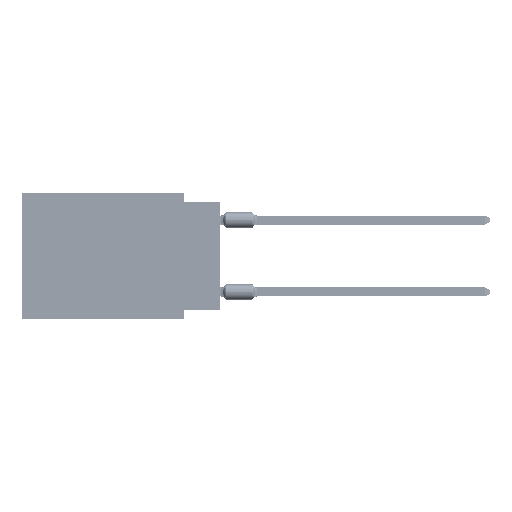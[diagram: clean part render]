
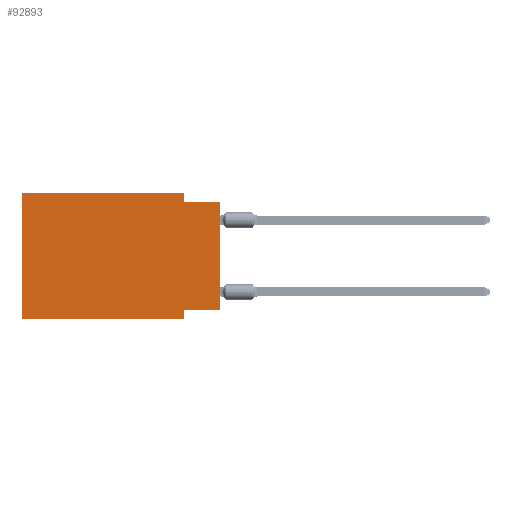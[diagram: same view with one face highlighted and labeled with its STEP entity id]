
A CAD part, left-side view. The second image highlights one B-rep face of the part: STEP entity #92893.
In plain terms, the highlighted planar face has unit normal (-1, 0, 0).
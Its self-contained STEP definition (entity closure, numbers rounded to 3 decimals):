
#2600 = CARTESIAN_POINT ( 'NONE',  ( 0., 0., -8.255 ) ) ;
#4311 = DIRECTION ( 'NONE',  ( 0., -1., 0. ) ) ;
#6535 = CARTESIAN_POINT ( 'NONE',  ( 0., 0., -0.635 ) ) ;
#6693 = CARTESIAN_POINT ( 'NONE',  ( 0., 0., 0. ) ) ;
#10922 = DIRECTION ( 'NONE',  ( 0., 0., -1. ) ) ;
#11883 = CARTESIAN_POINT ( 'NONE',  ( 0., 13.97, 0. ) ) ;
#12060 = FACE_OUTER_BOUND ( 'NONE', #67928, .T. ) ;
#13523 = DIRECTION ( 'NONE',  ( 0., 0., -1. ) ) ;
#13532 = EDGE_CURVE ( 'NONE', #15700, #110712, #107723, .T. ) ;
#14979 = LINE ( 'NONE', #6693, #100737 ) ;
#15146 = CARTESIAN_POINT ( 'NONE',  ( 0., 13.97, -8.89 ) ) ;
#15330 = CARTESIAN_POINT ( 'NONE',  ( 0., 2.54, -0.635 ) ) ;
#15700 = VERTEX_POINT ( 'NONE', #2600 ) ;
#16243 = CARTESIAN_POINT ( 'NONE',  ( 0., 0., -0.635 ) ) ;
#17698 = DIRECTION ( 'NONE',  ( 0., 1., 0. ) ) ;
#19477 = EDGE_CURVE ( 'NONE', #15700, #97066, #14979, .T. ) ;
#24214 = ORIENTED_EDGE ( 'NONE', *, *, #30494, .F. ) ;
#24702 = VECTOR ( 'NONE', #115147, 1000. ) ;
#26318 = EDGE_CURVE ( 'NONE', #110712, #85027, #102392, .T. ) ;
#27776 = CARTESIAN_POINT ( 'NONE',  ( 0., 2.54, -8.255 ) ) ;
#30494 = EDGE_CURVE ( 'NONE', #88601, #97066, #116302, .T. ) ;
#31571 = VECTOR ( 'NONE', #17698, 1000. ) ;
#32528 = VECTOR ( 'NONE', #65891, 1000. ) ;
#35267 = ORIENTED_EDGE ( 'NONE', *, *, #13532, .F. ) ;
#35494 = ORIENTED_EDGE ( 'NONE', *, *, #26318, .F. ) ;
#39331 = ORIENTED_EDGE ( 'NONE', *, *, #19477, .T. ) ;
#39921 = ORIENTED_EDGE ( 'NONE', *, *, #89007, .F. ) ;
#47259 = ORIENTED_EDGE ( 'NONE', *, *, #64930, .F. ) ;
#51095 = LINE ( 'NONE', #58796, #94188 ) ;
#51904 = CARTESIAN_POINT ( 'NONE',  ( 0., 13.97, 0. ) ) ;
#53016 = LINE ( 'NONE', #114642, #76101 ) ;
#55259 = LINE ( 'NONE', #92558, #32528 ) ;
#56649 = VERTEX_POINT ( 'NONE', #15146 ) ;
#58796 = CARTESIAN_POINT ( 'NONE',  ( 0., 13.97, 0. ) ) ;
#59113 = ORIENTED_EDGE ( 'NONE', *, *, #72431, .F. ) ;
#62697 = CARTESIAN_POINT ( 'NONE',  ( 0., 0., -8.255 ) ) ;
#64098 = VECTOR ( 'NONE', #96910, 1000. ) ;
#64930 = EDGE_CURVE ( 'NONE', #73414, #88601, #53016, .T. ) ;
#65891 = DIRECTION ( 'NONE',  ( 0., -1., 0. ) ) ;
#65936 = PLANE ( 'NONE',  #66433 ) ;
#66433 = AXIS2_PLACEMENT_3D ( 'NONE', #84309, #92033, #10922 ) ;
#67928 = EDGE_LOOP ( 'NONE', ( #39331, #24214, #47259, #59113, #39921, #68480, #35494, #35267 ) ) ;
#68480 = ORIENTED_EDGE ( 'NONE', *, *, #94149, .T. ) ;
#72431 = EDGE_CURVE ( 'NONE', #78267, #73414, #51095, .T. ) ;
#73414 = VERTEX_POINT ( 'NONE', #107616 ) ;
#76101 = VECTOR ( 'NONE', #79657, 1000. ) ;
#77936 = LINE ( 'NONE', #51904, #64098 ) ;
#78267 = VERTEX_POINT ( 'NONE', #11883 ) ;
#79657 = DIRECTION ( 'NONE',  ( 0., 0., -1. ) ) ;
#82636 = VECTOR ( 'NONE', #13523, 1000. ) ;
#84309 = CARTESIAN_POINT ( 'NONE',  ( 0., 13.97, 0. ) ) ;
#85027 = VERTEX_POINT ( 'NONE', #103198 ) ;
#88413 = DIRECTION ( 'NONE',  ( 0., 0., 1. ) ) ;
#88601 = VERTEX_POINT ( 'NONE', #15330 ) ;
#89007 = EDGE_CURVE ( 'NONE', #56649, #78267, #77936, .T. ) ;
#92033 = DIRECTION ( 'NONE',  ( 1., 0., 0. ) ) ;
#92558 = CARTESIAN_POINT ( 'NONE',  ( 0., 13.97, -8.89 ) ) ;
#92893 = ADVANCED_FACE ( 'NONE', ( #12060 ), #65936, .F. ) ;
#94149 = EDGE_CURVE ( 'NONE', #56649, #85027, #55259, .T. ) ;
#94188 = VECTOR ( 'NONE', #4311, 1000. ) ;
#94661 = CARTESIAN_POINT ( 'NONE',  ( 0., 2.54, -8.89 ) ) ;
#96910 = DIRECTION ( 'NONE',  ( 0., 0., 1. ) ) ;
#97066 = VERTEX_POINT ( 'NONE', #6535 ) ;
#100737 = VECTOR ( 'NONE', #88413, 1000. ) ;
#102392 = LINE ( 'NONE', #94661, #82636 ) ;
#103198 = CARTESIAN_POINT ( 'NONE',  ( 0., 2.54, -8.89 ) ) ;
#107616 = CARTESIAN_POINT ( 'NONE',  ( 0., 2.54, 0. ) ) ;
#107723 = LINE ( 'NONE', #62697, #31571 ) ;
#110712 = VERTEX_POINT ( 'NONE', #27776 ) ;
#114642 = CARTESIAN_POINT ( 'NONE',  ( 0., 2.54, 0. ) ) ;
#115147 = DIRECTION ( 'NONE',  ( 0., -1., 0. ) ) ;
#116302 = LINE ( 'NONE', #16243, #24702 ) ;
